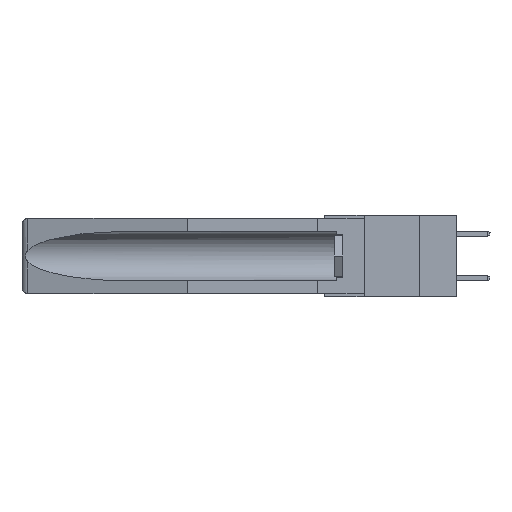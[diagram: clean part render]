
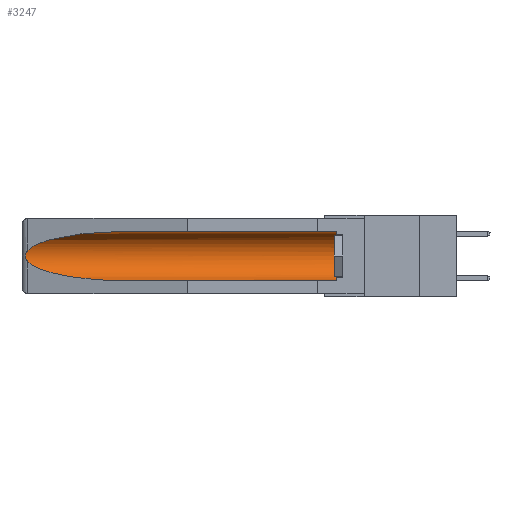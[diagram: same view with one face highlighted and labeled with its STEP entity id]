
A CAD part, left-side view. The second image highlights one B-rep face of the part: STEP entity #3247.
In plain terms, the highlighted cylindrical face has radius 2.857 mm (diameter 5.715 mm), a partial arc.
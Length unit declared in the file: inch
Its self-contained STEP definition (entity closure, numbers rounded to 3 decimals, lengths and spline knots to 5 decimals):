
#1054 = EDGE_LOOP ( 'NONE', ( #1852, #20892, #2805, #1313, #10327, #11124 ) ) ;
#1313 = ORIENTED_EDGE ( 'NONE', *, *, #5812, .F. ) ;
#1852 = ORIENTED_EDGE ( 'NONE', *, *, #10874, .T. ) ;
#2101 = CARTESIAN_POINT ( 'NONE',  ( 0.26537, 1.52718, -0.14972 ) ) ;
#2805 = ORIENTED_EDGE ( 'NONE', *, *, #10166, .T. ) ;
#2970 =( BOUNDED_CURVE ( )  B_SPLINE_CURVE ( 3, ( #19825, #23666, #11989, #2101 ),
 .UNSPECIFIED., .F., .F. ) 
 B_SPLINE_CURVE_WITH_KNOTS ( ( 4, 4 ),
 ( 4.71239, 6.08839 ),
 .UNSPECIFIED. ) 
 CURVE ( )  GEOMETRIC_REPRESENTATION_ITEM ( )  RATIONAL_B_SPLINE_CURVE ( ( 1., 0.848, 0.848, 1. ) ) 
 REPRESENTATION_ITEM ( '' )  );
#3042 = DIRECTION ( 'NONE',  ( 0., 0., 1. ) ) ;
#3226 = CARTESIAN_POINT ( 'NONE',  ( 0.2675, 1.53308, -0.17534 ) ) ;
#3247 = ADVANCED_FACE ( 'NONE', ( #24907 ), #5255, .F. ) ;
#3776 = CARTESIAN_POINT ( 'NONE',  ( 0.155, -0.30754, -0.284 ) ) ;
#5237 = CARTESIAN_POINT ( 'NONE',  ( 0.26654, 1.53092, -0.15636 ) ) ;
#5255 = CYLINDRICAL_SURFACE ( 'NONE', #9270, 0.1125 ) ;
#5315 = DIRECTION ( 'NONE',  ( 0., -1., 0. ) ) ;
#5326 = CARTESIAN_POINT ( 'NONE',  ( 0.2675, 1.53308, -0.16763 ) ) ;
#5812 = EDGE_CURVE ( 'NONE', #17603, #20423, #22361, .T. ) ;
#7245 = CARTESIAN_POINT ( 'NONE',  ( 0.26537, 1.52718, -0.14972 ) ) ;
#7255 = CIRCLE ( 'NONE', #17770, 0.1125 ) ;
#7273 = CARTESIAN_POINT ( 'NONE',  ( 0.21114, 1.30732, -0.284 ) ) ;
#7357 = CARTESIAN_POINT ( 'NONE',  ( 0.26537, 1.52718, -0.19328 ) ) ;
#7425 = CARTESIAN_POINT ( 'NONE',  ( 0.26537, 1.52718, -0.19328 ) ) ;
#7622 =( BOUNDED_CURVE ( )  B_SPLINE_CURVE ( 3, ( #7357, #9348, #7273, #11317 ),
 .UNSPECIFIED., .F., .F. ) 
 B_SPLINE_CURVE_WITH_KNOTS ( ( 4, 4 ),
 ( 0.1948, 1.5708 ),
 .UNSPECIFIED. ) 
 CURVE ( )  GEOMETRIC_REPRESENTATION_ITEM ( )  RATIONAL_B_SPLINE_CURVE ( ( 1., 0.848, 0.848, 1. ) ) 
 REPRESENTATION_ITEM ( '' )  );
#8512 = VECTOR ( 'NONE', #17119, 39.37008 ) ;
#8783 = CARTESIAN_POINT ( 'NONE',  ( 0.155, 0.126, -0.059 ) ) ;
#9167 = CARTESIAN_POINT ( 'NONE',  ( 0.155, -0.30754, -0.059 ) ) ;
#9210 = VECTOR ( 'NONE', #25076, 39.37008 ) ;
#9238 = CARTESIAN_POINT ( 'NONE',  ( 0.26597, 1.52961, -0.15275 ) ) ;
#9270 = AXIS2_PLACEMENT_3D ( 'NONE', #13739, #23534, #19684 ) ;
#9348 = CARTESIAN_POINT ( 'NONE',  ( 0.25451, 1.48313, -0.24835 ) ) ;
#9615 = CARTESIAN_POINT ( 'NONE',  ( 0.155, 1.07973, -0.059 ) ) ;
#10166 = EDGE_CURVE ( 'NONE', #19791, #20423, #7622, .T. ) ;
#10200 = EDGE_CURVE ( 'NONE', #12132, #17615, #17069, .T. ) ;
#10327 = ORIENTED_EDGE ( 'NONE', *, *, #22431, .T. ) ;
#10874 = EDGE_CURVE ( 'NONE', #17615, #23461, #2970, .T. ) ;
#11124 = ORIENTED_EDGE ( 'NONE', *, *, #10200, .T. ) ;
#11317 = CARTESIAN_POINT ( 'NONE',  ( 0.155, 1.07973, -0.284 ) ) ;
#11989 = CARTESIAN_POINT ( 'NONE',  ( 0.25451, 1.48313, -0.09465 ) ) ;
#12132 = VERTEX_POINT ( 'NONE', #8783 ) ;
#13003 = CARTESIAN_POINT ( 'NONE',  ( 0.155, 0.126, -0.1715 ) ) ;
#13071 = CARTESIAN_POINT ( 'NONE',  ( 0.26537, 1.52718, -0.14972 ) ) ;
#13739 = CARTESIAN_POINT ( 'NONE',  ( 0.155, -0.30754, -0.1715 ) ) ;
#13742 = CARTESIAN_POINT ( 'NONE',  ( 0.155, 0.126, -0.284 ) ) ;
#15062 = CARTESIAN_POINT ( 'NONE',  ( 0.2673, 1.5327, -0.16383 ) ) ;
#16230 = EDGE_CURVE ( 'NONE', #23461, #19791, #25379, .T. ) ;
#16843 = CARTESIAN_POINT ( 'NONE',  ( 0.155, 1.07973, -0.284 ) ) ;
#17069 = LINE ( 'NONE', #9167, #8512 ) ;
#17119 = DIRECTION ( 'NONE',  ( 0., 1., 0. ) ) ;
#17354 = CARTESIAN_POINT ( 'NONE',  ( 0.26597, 1.5296, -0.19026 ) ) ;
#17603 = VERTEX_POINT ( 'NONE', #13742 ) ;
#17615 = VERTEX_POINT ( 'NONE', #9615 ) ;
#17770 = AXIS2_PLACEMENT_3D ( 'NONE', #13003, #5315, #3042 ) ;
#18974 = CARTESIAN_POINT ( 'NONE',  ( 0.26655, 1.53094, -0.18657 ) ) ;
#19684 = DIRECTION ( 'NONE',  ( 0., 0., 1. ) ) ;
#19791 = VERTEX_POINT ( 'NONE', #22843 ) ;
#19825 = CARTESIAN_POINT ( 'NONE',  ( 0.155, 1.07973, -0.059 ) ) ;
#20423 = VERTEX_POINT ( 'NONE', #16843 ) ;
#20892 = ORIENTED_EDGE ( 'NONE', *, *, #16230, .T. ) ;
#20940 = CARTESIAN_POINT ( 'NONE',  ( 0.2673, 1.53269, -0.17917 ) ) ;
#22361 = LINE ( 'NONE', #3776, #9210 ) ;
#22431 = EDGE_CURVE ( 'NONE', #17603, #12132, #7255, .T. ) ;
#22843 = CARTESIAN_POINT ( 'NONE',  ( 0.26537, 1.52718, -0.19328 ) ) ;
#23461 = VERTEX_POINT ( 'NONE', #13071 ) ;
#23534 = DIRECTION ( 'NONE',  ( 0., 1., 0. ) ) ;
#23666 = CARTESIAN_POINT ( 'NONE',  ( 0.21114, 1.30732, -0.059 ) ) ;
#24907 = FACE_OUTER_BOUND ( 'NONE', #1054, .T. ) ;
#25076 = DIRECTION ( 'NONE',  ( 0., 1., 0. ) ) ;
#25379 = B_SPLINE_CURVE_WITH_KNOTS ( 'NONE', 3,
 ( #7245, #9238, #5237, #15062, #5326, #3226, #20940, #18974, #17354, #7425 ),
 .UNSPECIFIED., .F., .F.,
 ( 4, 2, 2, 2, 4 ),
 ( 0., 0.00029, 0.00058, 0.00087, 0.00117 ),
 .UNSPECIFIED. ) ;
